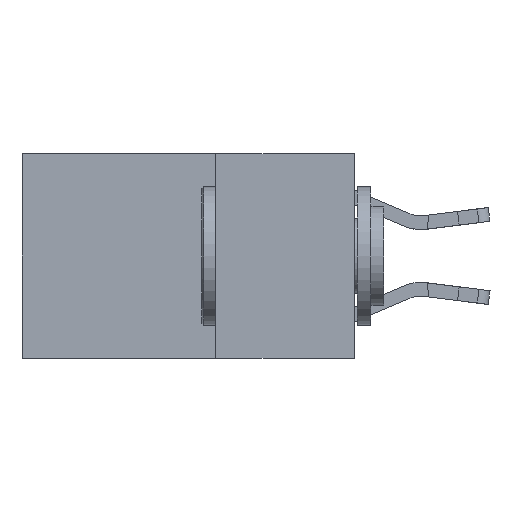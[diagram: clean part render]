
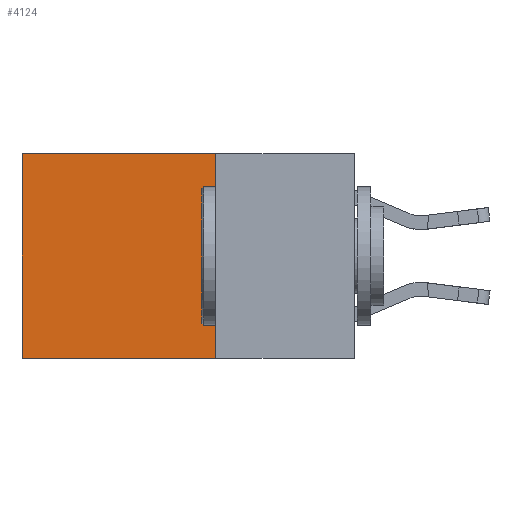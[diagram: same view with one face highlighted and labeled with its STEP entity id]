
A CAD part, left-side view. The second image highlights one B-rep face of the part: STEP entity #4124.
In plain terms, the highlighted planar face has unit normal (-1, 0, 0).
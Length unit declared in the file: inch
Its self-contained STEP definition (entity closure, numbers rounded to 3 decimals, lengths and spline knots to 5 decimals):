
#877 = DIRECTION ( 'NONE',  ( 0., 0., -1. ) ) ;
#1361 = CARTESIAN_POINT ( 'NONE',  ( 0.2625, 0.6, 0. ) ) ;
#1914 = LINE ( 'NONE', #13941, #5764 ) ;
#2763 = VERTEX_POINT ( 'NONE', #9209 ) ;
#3281 = ORIENTED_EDGE ( 'NONE', *, *, #9934, .T. ) ;
#4084 = VERTEX_POINT ( 'NONE', #5982 ) ;
#4124 = ADVANCED_FACE ( 'NONE', ( #19211 ), #14210, .F. ) ;
#4881 = EDGE_CURVE ( 'NONE', #2763, #4084, #16020, .T. ) ;
#5388 = EDGE_CURVE ( 'NONE', #13377, #15149, #1914, .T. ) ;
#5738 = CARTESIAN_POINT ( 'NONE',  ( 0.2625, 0.25, 0. ) ) ;
#5764 = VECTOR ( 'NONE', #877, 39.37008 ) ;
#5982 = CARTESIAN_POINT ( 'NONE',  ( 0.2625, 0.6, -0.37 ) ) ;
#6052 = DIRECTION ( 'NONE',  ( 0., 0., -1. ) ) ;
#7678 = LINE ( 'NONE', #19883, #19106 ) ;
#8383 = EDGE_LOOP ( 'NONE', ( #14447, #19612, #15825, #3281 ) ) ;
#9209 = CARTESIAN_POINT ( 'NONE',  ( 0.2625, 0.6, 0. ) ) ;
#9934 = EDGE_CURVE ( 'NONE', #13377, #2763, #7678, .T. ) ;
#10353 = LINE ( 'NONE', #11300, #14688 ) ;
#11184 = VECTOR ( 'NONE', #12835, 39.37008 ) ;
#11300 = CARTESIAN_POINT ( 'NONE',  ( 0.2625, 0.25, -0.37 ) ) ;
#11905 = AXIS2_PLACEMENT_3D ( 'NONE', #12581, #15842, #6052 ) ;
#12304 = EDGE_CURVE ( 'NONE', #15149, #4084, #10353, .T. ) ;
#12414 = CARTESIAN_POINT ( 'NONE',  ( 0.2625, 0.25, -0.37 ) ) ;
#12581 = CARTESIAN_POINT ( 'NONE',  ( 0.2625, 0.25, 0. ) ) ;
#12835 = DIRECTION ( 'NONE',  ( 0., 0., -1. ) ) ;
#13377 = VERTEX_POINT ( 'NONE', #5738 ) ;
#13941 = CARTESIAN_POINT ( 'NONE',  ( 0.2625, 0.25, 0. ) ) ;
#14210 = PLANE ( 'NONE',  #11905 ) ;
#14447 = ORIENTED_EDGE ( 'NONE', *, *, #4881, .T. ) ;
#14688 = VECTOR ( 'NONE', #17751, 39.37008 ) ;
#15149 = VERTEX_POINT ( 'NONE', #12414 ) ;
#15825 = ORIENTED_EDGE ( 'NONE', *, *, #5388, .F. ) ;
#15842 = DIRECTION ( 'NONE',  ( 1., 0., 0. ) ) ;
#16020 = LINE ( 'NONE', #1361, #11184 ) ;
#16718 = DIRECTION ( 'NONE',  ( 0., 1., 0. ) ) ;
#17751 = DIRECTION ( 'NONE',  ( 0., 1., 0. ) ) ;
#19106 = VECTOR ( 'NONE', #16718, 39.37008 ) ;
#19211 = FACE_OUTER_BOUND ( 'NONE', #8383, .T. ) ;
#19612 = ORIENTED_EDGE ( 'NONE', *, *, #12304, .F. ) ;
#19883 = CARTESIAN_POINT ( 'NONE',  ( 0.2625, 0.25, 0. ) ) ;
